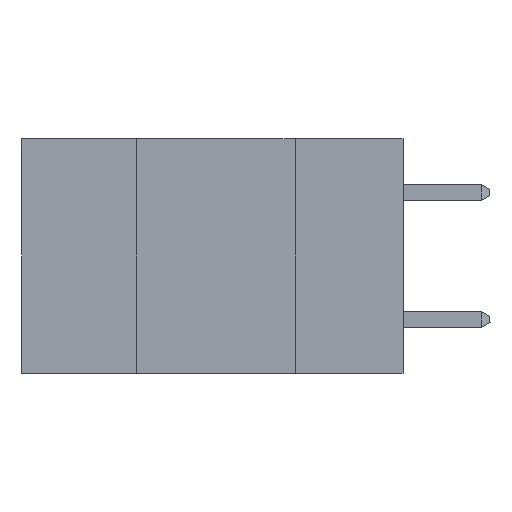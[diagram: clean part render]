
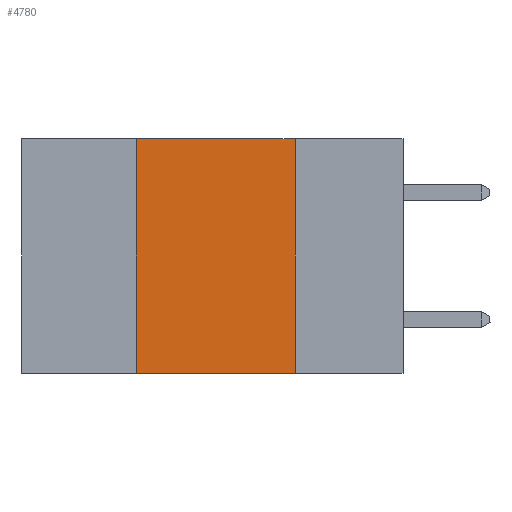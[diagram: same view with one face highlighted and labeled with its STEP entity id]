
A CAD part, left-side view. The second image highlights one B-rep face of the part: STEP entity #4780.
In plain terms, the highlighted planar face has unit normal (-1, 0, 0).
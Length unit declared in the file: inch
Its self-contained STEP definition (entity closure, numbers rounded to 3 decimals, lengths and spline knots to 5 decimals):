
#1349 = CARTESIAN_POINT ( 'NONE',  ( 0., 0.6, 0. ) ) ;
#1649 = VECTOR ( 'NONE', #16587, 39.37008 ) ;
#1972 = CARTESIAN_POINT ( 'NONE',  ( 0., 0.42, 0. ) ) ;
#2971 = DIRECTION ( 'NONE',  ( 0., -1., 0. ) ) ;
#3691 = CARTESIAN_POINT ( 'NONE',  ( 0., 0.17, 0. ) ) ;
#4422 = EDGE_CURVE ( 'NONE', #22833, #18050, #9083, .T. ) ;
#4780 = ADVANCED_FACE ( 'NONE', ( #6824 ), #19403, .F. ) ;
#5077 = DIRECTION ( 'NONE',  ( 0., 0., -1. ) ) ;
#5162 = ORIENTED_EDGE ( 'NONE', *, *, #19714, .F. ) ;
#5287 = VERTEX_POINT ( 'NONE', #9137 ) ;
#5781 = LINE ( 'NONE', #3691, #1649 ) ;
#5792 = EDGE_CURVE ( 'NONE', #5287, #18050, #5781, .T. ) ;
#6483 = VECTOR ( 'NONE', #7087, 39.37008 ) ;
#6824 = FACE_OUTER_BOUND ( 'NONE', #12907, .T. ) ;
#7087 = DIRECTION ( 'NONE',  ( 0., -1., 0. ) ) ;
#8733 = CARTESIAN_POINT ( 'NONE',  ( 0., 0.17, -0.37 ) ) ;
#8876 = CARTESIAN_POINT ( 'NONE',  ( 0., 0.42, -0.37 ) ) ;
#9083 = LINE ( 'NONE', #14697, #6483 ) ;
#9137 = CARTESIAN_POINT ( 'NONE',  ( 0., 0.17, 0. ) ) ;
#11345 = ORIENTED_EDGE ( 'NONE', *, *, #5792, .F. ) ;
#11552 = EDGE_CURVE ( 'NONE', #16199, #5287, #15531, .T. ) ;
#12907 = EDGE_LOOP ( 'NONE', ( #11345, #20048, #5162, #13961 ) ) ;
#13961 = ORIENTED_EDGE ( 'NONE', *, *, #4422, .T. ) ;
#14697 = CARTESIAN_POINT ( 'NONE',  ( 0., 0.6, -0.37 ) ) ;
#15531 = LINE ( 'NONE', #15646, #15673 ) ;
#15627 = DIRECTION ( 'NONE',  ( 1., 0., 0. ) ) ;
#15646 = CARTESIAN_POINT ( 'NONE',  ( 0., 0.6, 0. ) ) ;
#15673 = VECTOR ( 'NONE', #2971, 39.37008 ) ;
#16131 = CARTESIAN_POINT ( 'NONE',  ( 0., 0.42, 0. ) ) ;
#16199 = VERTEX_POINT ( 'NONE', #1972 ) ;
#16257 = LINE ( 'NONE', #16131, #18823 ) ;
#16587 = DIRECTION ( 'NONE',  ( 0., 0., -1. ) ) ;
#18050 = VERTEX_POINT ( 'NONE', #8733 ) ;
#18823 = VECTOR ( 'NONE', #22942, 39.37008 ) ;
#19403 = PLANE ( 'NONE',  #20751 ) ;
#19714 = EDGE_CURVE ( 'NONE', #22833, #16199, #16257, .T. ) ;
#20048 = ORIENTED_EDGE ( 'NONE', *, *, #11552, .F. ) ;
#20751 = AXIS2_PLACEMENT_3D ( 'NONE', #1349, #15627, #5077 ) ;
#22833 = VERTEX_POINT ( 'NONE', #8876 ) ;
#22942 = DIRECTION ( 'NONE',  ( 0., 0., 1. ) ) ;
